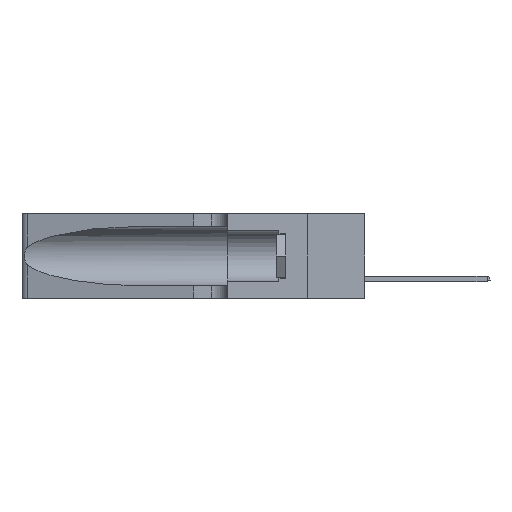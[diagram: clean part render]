
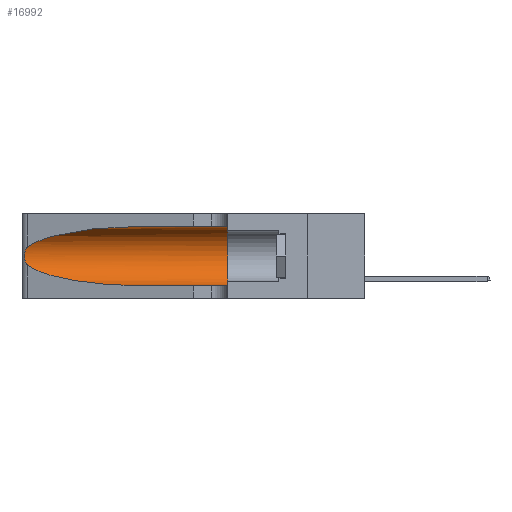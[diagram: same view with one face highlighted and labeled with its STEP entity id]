
A CAD part, left-side view. The second image highlights one B-rep face of the part: STEP entity #16992.
In plain terms, the highlighted cylindrical face has radius 3.308 mm (diameter 6.617 mm), a partial arc.
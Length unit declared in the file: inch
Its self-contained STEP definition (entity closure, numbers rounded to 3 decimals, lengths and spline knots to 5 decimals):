
#467 = CARTESIAN_POINT ( 'NONE',  ( 0.25856, 1.23593, 0.16098 ) ) ;
#673 = VECTOR ( 'NONE', #21927, 39.37008 ) ;
#773 = DIRECTION ( 'NONE',  ( 0., 0., 1. ) ) ;
#844 = AXIS2_PLACEMENT_3D ( 'NONE', #24025, #18053, #22177 ) ;
#1312 = LINE ( 'NONE', #25912, #673 ) ;
#1662 = VERTEX_POINT ( 'NONE', #2991 ) ;
#1933 = AXIS2_PLACEMENT_3D ( 'NONE', #20900, #2835, #773 ) ;
#2518 = ORIENTED_EDGE ( 'NONE', *, *, #18151, .F. ) ;
#2621 = CARTESIAN_POINT ( 'NONE',  ( 0.26075, 1.23896, 0.178 ) ) ;
#2835 = DIRECTION ( 'NONE',  ( 0., 1., 0. ) ) ;
#2991 = CARTESIAN_POINT ( 'NONE',  ( 0.25487, 1.22718, 0.22369 ) ) ;
#3063 = CARTESIAN_POINT ( 'NONE',  ( 0.25487, 1.22718, 0.14631 ) ) ;
#3444 = ORIENTED_EDGE ( 'NONE', *, *, #12842, .T. ) ;
#4505 = EDGE_LOOP ( 'NONE', ( #18928, #13370, #3444, #15377, #19054, #2518 ) ) ;
#4869 = CARTESIAN_POINT ( 'NONE',  ( 0.18966, 0.96281, 0.05475 ) ) ;
#5001 = CARTESIAN_POINT ( 'NONE',  ( 0.1305, 0.72297, 0.31525 ) ) ;
#6123 = CARTESIAN_POINT ( 'NONE',  ( 0.25639, 1.23184, 0.21858 ) ) ;
#6300 = CARTESIAN_POINT ( 'NONE',  ( 0.1305, 0.35, 0.31525 ) ) ;
#6312 = LINE ( 'NONE', #16023, #22875 ) ;
#6482 = VERTEX_POINT ( 'NONE', #9767 ) ;
#6507 = FACE_OUTER_BOUND ( 'NONE', #4505, .T. ) ;
#6649 = CARTESIAN_POINT ( 'NONE',  ( 0.25789, 1.23486, 0.15765 ) ) ;
#6776 = CARTESIAN_POINT ( 'NONE',  ( 0.25487, 1.22718, 0.22369 ) ) ;
#6828 = CARTESIAN_POINT ( 'NONE',  ( 0.2373, 1.15595, 0.08982 ) ) ;
#6855 = CYLINDRICAL_SURFACE ( 'NONE', #844, 0.13025 ) ;
#6926 = CARTESIAN_POINT ( 'NONE',  ( 0.1305, 0.35, 0.05475 ) ) ;
#7221 = CARTESIAN_POINT ( 'NONE',  ( 0.25487, 1.22718, 0.14631 ) ) ;
#7938 = CARTESIAN_POINT ( 'NONE',  ( 0.25555, 1.22994, 0.2215 ) ) ;
#9058 = CARTESIAN_POINT ( 'NONE',  ( 0.25639, 1.23186, 0.15144 ) ) ;
#9767 = CARTESIAN_POINT ( 'NONE',  ( 0.25487, 1.22718, 0.14631 ) ) ;
#10065 = CARTESIAN_POINT ( 'NONE',  ( 0.25787, 1.23484, 0.2124 ) ) ;
#11934 = EDGE_CURVE ( 'NONE', #1662, #6482, #21030, .T. ) ;
#12534 = DIRECTION ( 'NONE',  ( 0., -1., 0. ) ) ;
#12779 = CIRCLE ( 'NONE', #1933, 0.13025 ) ;
#12842 = EDGE_CURVE ( 'NONE', #6482, #21066, #26245, .T. ) ;
#12864 = CARTESIAN_POINT ( 'NONE',  ( 0.1305, 0.72297, 0.05475 ) ) ;
#13233 = CARTESIAN_POINT ( 'NONE',  ( 0.25555, 1.22993, 0.14849 ) ) ;
#13370 = ORIENTED_EDGE ( 'NONE', *, *, #11934, .T. ) ;
#14156 = EDGE_CURVE ( 'NONE', #21066, #23910, #6312, .T. ) ;
#14955 = CARTESIAN_POINT ( 'NONE',  ( 0.18966, 0.96281, 0.31525 ) ) ;
#15377 = ORIENTED_EDGE ( 'NONE', *, *, #14156, .T. ) ;
#16023 = CARTESIAN_POINT ( 'NONE',  ( 0.1305, 1.61858, 0.05475 ) ) ;
#16992 = ADVANCED_FACE ( 'NONE', ( #6507 ), #6855, .F. ) ;
#18053 = DIRECTION ( 'NONE',  ( 0., -1., 0. ) ) ;
#18151 = EDGE_CURVE ( 'NONE', #22664, #24110, #1312, .T. ) ;
#18922 = CARTESIAN_POINT ( 'NONE',  ( 0.2373, 1.15595, 0.28018 ) ) ;
#18928 = ORIENTED_EDGE ( 'NONE', *, *, #26143, .T. ) ;
#18991 = CARTESIAN_POINT ( 'NONE',  ( 0.26018, 1.23835, 0.19895 ) ) ;
#19054 = ORIENTED_EDGE ( 'NONE', *, *, #21502, .F. ) ;
#20330 = CARTESIAN_POINT ( 'NONE',  ( 0.25854, 1.2359, 0.20912 ) ) ;
#20900 = CARTESIAN_POINT ( 'NONE',  ( 0.1305, 0.35, 0.185 ) ) ;
#20999 = CARTESIAN_POINT ( 'NONE',  ( 0.1305, 0.72297, 0.31525 ) ) ;
#21030 = B_SPLINE_CURVE_WITH_KNOTS ( 'NONE', 3,
 ( #26066, #7938, #6123, #10065, #20330, #18991, #22762, #2621, #24867, #467, #6649, #9058, #13233, #7221 ),
 .UNSPECIFIED., .F., .F.,
 ( 4, 2, 2, 2, 2, 2, 4 ),
 ( 0., 0.00027, 0.00053, 0.00107, 0.0016, 0.00187, 0.00214 ),
 .UNSPECIFIED. ) ;
#21066 = VERTEX_POINT ( 'NONE', #12864 ) ;
#21502 = EDGE_CURVE ( 'NONE', #24110, #23910, #12779, .T. ) ;
#21513 =( BOUNDED_CURVE ( )  B_SPLINE_CURVE ( 3, ( #5001, #14955, #18922, #6776 ),
 .UNSPECIFIED., .F., .T. ) 
 B_SPLINE_CURVE_WITH_KNOTS ( ( 4, 4 ),
 ( 1.5708, 2.84003 ),
 .UNSPECIFIED. ) 
 CURVE ( )  GEOMETRIC_REPRESENTATION_ITEM ( )  RATIONAL_B_SPLINE_CURVE ( ( 1., 0.87, 0.87, 1. ) ) 
 REPRESENTATION_ITEM ( '' )  );
#21927 = DIRECTION ( 'NONE',  ( 0., -1., 0. ) ) ;
#22177 = DIRECTION ( 'NONE',  ( 0., 0., -1. ) ) ;
#22664 = VERTEX_POINT ( 'NONE', #20999 ) ;
#22762 = CARTESIAN_POINT ( 'NONE',  ( 0.26075, 1.23896, 0.19203 ) ) ;
#22875 = VECTOR ( 'NONE', #12534, 39.37008 ) ;
#23534 = CARTESIAN_POINT ( 'NONE',  ( 0.1305, 0.72297, 0.05475 ) ) ;
#23910 = VERTEX_POINT ( 'NONE', #6926 ) ;
#24025 = CARTESIAN_POINT ( 'NONE',  ( 0.1305, 1.61858, 0.185 ) ) ;
#24110 = VERTEX_POINT ( 'NONE', #6300 ) ;
#24867 = CARTESIAN_POINT ( 'NONE',  ( 0.26017, 1.23833, 0.17102 ) ) ;
#25912 = CARTESIAN_POINT ( 'NONE',  ( 0.1305, 1.61858, 0.31525 ) ) ;
#26066 = CARTESIAN_POINT ( 'NONE',  ( 0.25487, 1.22718, 0.22369 ) ) ;
#26143 = EDGE_CURVE ( 'NONE', #22664, #1662, #21513, .T. ) ;
#26245 =( BOUNDED_CURVE ( )  B_SPLINE_CURVE ( 3, ( #3063, #6828, #4869, #23534 ),
 .UNSPECIFIED., .F., .T. ) 
 B_SPLINE_CURVE_WITH_KNOTS ( ( 4, 4 ),
 ( 3.44316, 4.71239 ),
 .UNSPECIFIED. ) 
 CURVE ( )  GEOMETRIC_REPRESENTATION_ITEM ( )  RATIONAL_B_SPLINE_CURVE ( ( 1., 0.87, 0.87, 1. ) ) 
 REPRESENTATION_ITEM ( '' )  );
